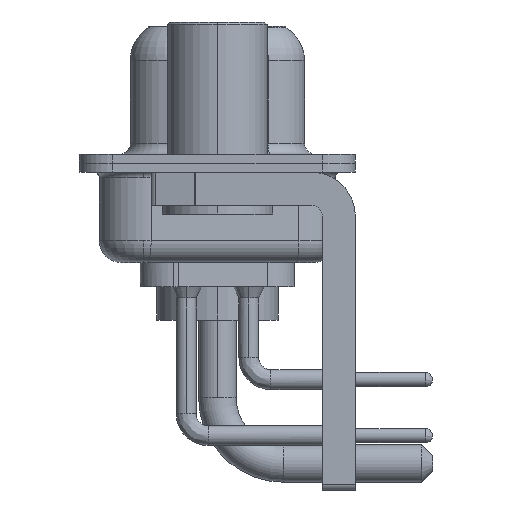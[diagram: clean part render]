
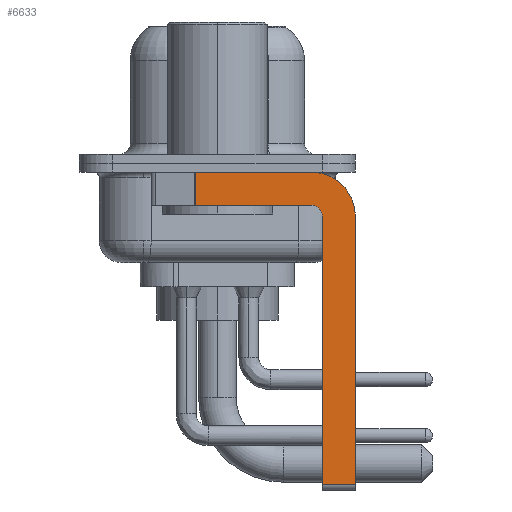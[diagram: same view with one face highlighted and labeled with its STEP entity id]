
A CAD part, left-side view. The second image highlights one B-rep face of the part: STEP entity #6633.
In plain terms, the highlighted planar face has unit normal (-1, 0, 0).
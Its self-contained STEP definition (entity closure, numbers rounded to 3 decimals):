
#195 = CARTESIAN_POINT ( 'NONE',  ( -2.9, -4.75, -14.8 ) ) ;
#915 = EDGE_CURVE ( 'NONE', #18080, #2018, #13208, .T. ) ;
#1095 = LINE ( 'NONE', #5024, #23300 ) ;
#1154 = ORIENTED_EDGE ( 'NONE', *, *, #19865, .F. ) ;
#1863 = LINE ( 'NONE', #195, #21527 ) ;
#1943 = VECTOR ( 'NONE', #20379, 1000. ) ;
#1996 = DIRECTION ( 'NONE',  ( 0., 0., 1. ) ) ;
#2018 = VERTEX_POINT ( 'NONE', #4944 ) ;
#2209 = ORIENTED_EDGE ( 'NONE', *, *, #6639, .F. ) ;
#3363 = EDGE_CURVE ( 'NONE', #18412, #11401, #25124, .T. ) ;
#3564 = VERTEX_POINT ( 'NONE', #9644 ) ;
#4490 = CARTESIAN_POINT ( 'NONE',  ( -2.9, -4.25, -2.4 ) ) ;
#4751 = CIRCLE ( 'NONE', #10449, 2. ) ;
#4944 = CARTESIAN_POINT ( 'NONE',  ( -2.9, -6.25, -14.55 ) ) ;
#5024 = CARTESIAN_POINT ( 'NONE',  ( -2.9, -6.25, -2.4 ) ) ;
#5481 = VECTOR ( 'NONE', #10702, 1000. ) ;
#5567 = EDGE_CURVE ( 'NONE', #3564, #20056, #6591, .T. ) ;
#5642 = CARTESIAN_POINT ( 'NONE',  ( -2.9, 0.978, -1.9 ) ) ;
#5982 = EDGE_CURVE ( 'NONE', #11778, #3564, #24343, .T. ) ;
#6591 = LINE ( 'NONE', #8378, #1943 ) ;
#6633 = ADVANCED_FACE ( 'NONE', ( #19465 ), #19331, .F. ) ;
#6639 = EDGE_CURVE ( 'NONE', #18080, #11778, #1863, .T. ) ;
#6763 = LINE ( 'NONE', #8558, #5481 ) ;
#7143 = VERTEX_POINT ( 'NONE', #17513 ) ;
#7566 = CARTESIAN_POINT ( 'NONE',  ( -2.9, -4.75, -14.55 ) ) ;
#7840 = DIRECTION ( 'NONE',  ( 1., 0., 0. ) ) ;
#8378 = CARTESIAN_POINT ( 'NONE',  ( -2.9, -4.25, -1.9 ) ) ;
#8440 = DIRECTION ( 'NONE',  ( -1., 0., 0. ) ) ;
#8558 = CARTESIAN_POINT ( 'NONE',  ( -2.9, 0.978, -1.9 ) ) ;
#8881 = AXIS2_PLACEMENT_3D ( 'NONE', #17665, #7840, #11915 ) ;
#9644 = CARTESIAN_POINT ( 'NONE',  ( -2.9, -4.25, -1.9 ) ) ;
#10096 = EDGE_CURVE ( 'NONE', #18412, #20056, #6763, .T. ) ;
#10107 = AXIS2_PLACEMENT_3D ( 'NONE', #4490, #8440, #16219 ) ;
#10449 = AXIS2_PLACEMENT_3D ( 'NONE', #16484, #18402, #16115 ) ;
#10702 = DIRECTION ( 'NONE',  ( 0., 0., -1. ) ) ;
#11401 = VERTEX_POINT ( 'NONE', #23135 ) ;
#11440 = DIRECTION ( 'NONE',  ( 0., -1., 0. ) ) ;
#11778 = VERTEX_POINT ( 'NONE', #13517 ) ;
#11915 = DIRECTION ( 'NONE',  ( 0., 0., -1. ) ) ;
#12788 = DIRECTION ( 'NONE',  ( 0., 0., -1. ) ) ;
#13208 = LINE ( 'NONE', #19100, #13311 ) ;
#13311 = VECTOR ( 'NONE', #11440, 1000. ) ;
#13517 = CARTESIAN_POINT ( 'NONE',  ( -2.9, -4.75, -2.4 ) ) ;
#13622 = VECTOR ( 'NONE', #17504, 1000. ) ;
#14282 = EDGE_CURVE ( 'NONE', #7143, #2018, #1095, .T. ) ;
#15454 = CARTESIAN_POINT ( 'NONE',  ( -2.9, 3., -0.4 ) ) ;
#15797 = EDGE_LOOP ( 'NONE', ( #16743, #17389, #17943, #19172, #2209, #25136, #22992, #1154 ) ) ;
#16115 = DIRECTION ( 'NONE',  ( 0., 0., -1. ) ) ;
#16219 = DIRECTION ( 'NONE',  ( 0., 0., 1. ) ) ;
#16484 = CARTESIAN_POINT ( 'NONE',  ( -2.9, -4.25, -2.4 ) ) ;
#16743 = ORIENTED_EDGE ( 'NONE', *, *, #3363, .F. ) ;
#17389 = ORIENTED_EDGE ( 'NONE', *, *, #10096, .T. ) ;
#17504 = DIRECTION ( 'NONE',  ( 0., -1., 0. ) ) ;
#17513 = CARTESIAN_POINT ( 'NONE',  ( -2.9, -6.25, -2.4 ) ) ;
#17665 = CARTESIAN_POINT ( 'NONE',  ( -2.9, -4.25, -2.4 ) ) ;
#17943 = ORIENTED_EDGE ( 'NONE', *, *, #5567, .F. ) ;
#18080 = VERTEX_POINT ( 'NONE', #7566 ) ;
#18402 = DIRECTION ( 'NONE',  ( 1., 0., 0. ) ) ;
#18412 = VERTEX_POINT ( 'NONE', #19623 ) ;
#19100 = CARTESIAN_POINT ( 'NONE',  ( -2.9, -4.25, -14.55 ) ) ;
#19172 = ORIENTED_EDGE ( 'NONE', *, *, #5982, .F. ) ;
#19331 = PLANE ( 'NONE',  #8881 ) ;
#19465 = FACE_OUTER_BOUND ( 'NONE', #15797, .T. ) ;
#19623 = CARTESIAN_POINT ( 'NONE',  ( -2.9, 0.978, -0.4 ) ) ;
#19865 = EDGE_CURVE ( 'NONE', #11401, #7143, #4751, .T. ) ;
#20056 = VERTEX_POINT ( 'NONE', #5642 ) ;
#20379 = DIRECTION ( 'NONE',  ( 0., 1., 0. ) ) ;
#21527 = VECTOR ( 'NONE', #1996, 1000. ) ;
#22992 = ORIENTED_EDGE ( 'NONE', *, *, #14282, .F. ) ;
#23135 = CARTESIAN_POINT ( 'NONE',  ( -2.9, -4.25, -0.4 ) ) ;
#23300 = VECTOR ( 'NONE', #12788, 1000. ) ;
#24343 = CIRCLE ( 'NONE', #10107, 0.5 ) ;
#25124 = LINE ( 'NONE', #15454, #13622 ) ;
#25136 = ORIENTED_EDGE ( 'NONE', *, *, #915, .T. ) ;
